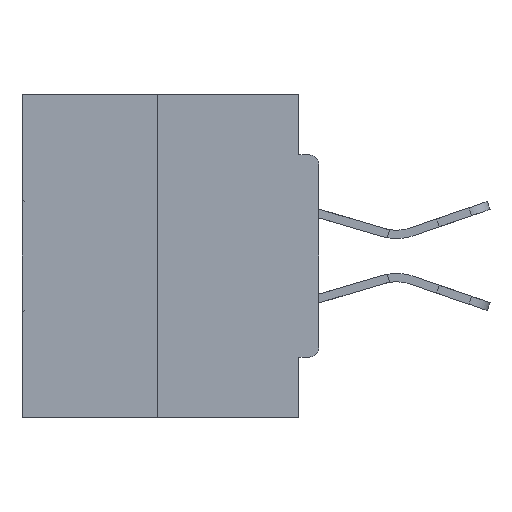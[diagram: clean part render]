
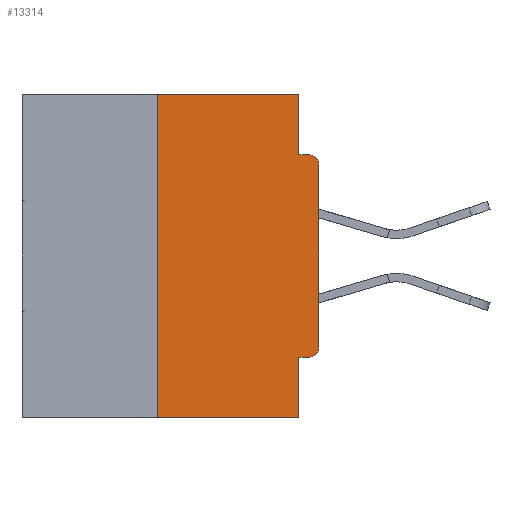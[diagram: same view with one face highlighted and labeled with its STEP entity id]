
A CAD part, left-side view. The second image highlights one B-rep face of the part: STEP entity #13314.
In plain terms, the highlighted planar face has unit normal (-1, 0, 0).
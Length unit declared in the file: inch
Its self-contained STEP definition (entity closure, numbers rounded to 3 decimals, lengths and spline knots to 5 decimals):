
#20 = PLANE ( 'NONE',  #43346 ) ;
#307 = CARTESIAN_POINT ( 'NONE',  ( 0., 0., -0.1085 ) ) ;
#514 = CARTESIAN_POINT ( 'NONE',  ( 0., 0.031, -0.4065 ) ) ;
#758 = ORIENTED_EDGE ( 'NONE', *, *, #14378, .F. ) ;
#1119 = VERTEX_POINT ( 'NONE', #307 ) ;
#1191 = EDGE_CURVE ( 'NONE', #15538, #8642, #17899, .T. ) ;
#1351 = LINE ( 'NONE', #39865, #3982 ) ;
#1389 = CARTESIAN_POINT ( 'NONE',  ( 0., 0.031, 0. ) ) ;
#2072 = LINE ( 'NONE', #3896, #15142 ) ;
#3095 = VECTOR ( 'NONE', #6852, 39.37008 ) ;
#3896 = CARTESIAN_POINT ( 'NONE',  ( 0., 0., -0.4065 ) ) ;
#3982 = VECTOR ( 'NONE', #26684, 39.37008 ) ;
#5141 = FACE_OUTER_BOUND ( 'NONE', #34798, .T. ) ;
#5734 = ORIENTED_EDGE ( 'NONE', *, *, #24932, .T. ) ;
#5832 = LINE ( 'NONE', #37845, #40338 ) ;
#6600 = CARTESIAN_POINT ( 'NONE',  ( 0., 0.031, -0.0935 ) ) ;
#6852 = DIRECTION ( 'NONE',  ( 0., 0., 1. ) ) ;
#8642 = VERTEX_POINT ( 'NONE', #16960 ) ;
#9210 = ORIENTED_EDGE ( 'NONE', *, *, #31386, .F. ) ;
#9304 = CARTESIAN_POINT ( 'NONE',  ( 0., 0., -0.0935 ) ) ;
#11231 = DIRECTION ( 'NONE',  ( 0., 0., -1. ) ) ;
#12776 = EDGE_CURVE ( 'NONE', #22746, #1119, #30275, .T. ) ;
#13314 = ADVANCED_FACE ( 'NONE', ( #5141 ), #20, .F. ) ;
#13691 = LINE ( 'NONE', #14069, #20993 ) ;
#14069 = CARTESIAN_POINT ( 'NONE',  ( 0., 0.25, 0. ) ) ;
#14216 = CARTESIAN_POINT ( 'NONE',  ( 0., 0.015, -0.4065 ) ) ;
#14378 = EDGE_CURVE ( 'NONE', #21782, #18243, #1351, .T. ) ;
#15142 = VECTOR ( 'NONE', #37388, 39.37008 ) ;
#15211 = CARTESIAN_POINT ( 'NONE',  ( 0., 0.25, -0.5 ) ) ;
#15538 = VERTEX_POINT ( 'NONE', #15211 ) ;
#15846 = ORIENTED_EDGE ( 'NONE', *, *, #1191, .T. ) ;
#15968 = CARTESIAN_POINT ( 'NONE',  ( 0., 0.015, -0.3915 ) ) ;
#16436 = CARTESIAN_POINT ( 'NONE',  ( 0., 0.015, -0.1085 ) ) ;
#16960 = CARTESIAN_POINT ( 'NONE',  ( 0., 0.031, -0.5 ) ) ;
#17398 = DIRECTION ( 'NONE',  ( 0., 0., 1. ) ) ;
#17876 = ORIENTED_EDGE ( 'NONE', *, *, #18327, .F. ) ;
#17899 = LINE ( 'NONE', #40274, #33579 ) ;
#18243 = VERTEX_POINT ( 'NONE', #41948 ) ;
#18327 = EDGE_CURVE ( 'NONE', #23149, #32677, #31568, .T. ) ;
#19325 = DIRECTION ( 'NONE',  ( -1., 0., 0. ) ) ;
#19808 = DIRECTION ( 'NONE',  ( 0., 0., -1. ) ) ;
#20993 = VECTOR ( 'NONE', #17398, 39.37008 ) ;
#21192 = CARTESIAN_POINT ( 'NONE',  ( 0., 0.25, 0. ) ) ;
#21782 = VERTEX_POINT ( 'NONE', #21192 ) ;
#22010 = AXIS2_PLACEMENT_3D ( 'NONE', #16436, #35870, #36016 ) ;
#22607 = CARTESIAN_POINT ( 'NONE',  ( 0., 0., 0. ) ) ;
#22614 = VECTOR ( 'NONE', #32389, 39.37008 ) ;
#22663 = DIRECTION ( 'NONE',  ( 0., 0., -1. ) ) ;
#22746 = VERTEX_POINT ( 'NONE', #40849 ) ;
#23149 = VERTEX_POINT ( 'NONE', #6600 ) ;
#24032 = ORIENTED_EDGE ( 'NONE', *, *, #43118, .F. ) ;
#24269 = ORIENTED_EDGE ( 'NONE', *, *, #26075, .F. ) ;
#24932 = EDGE_CURVE ( 'NONE', #30819, #22746, #27378, .T. ) ;
#26075 = EDGE_CURVE ( 'NONE', #15538, #21782, #13691, .T. ) ;
#26552 = AXIS2_PLACEMENT_3D ( 'NONE', #15968, #19325, #22663 ) ;
#26684 = DIRECTION ( 'NONE',  ( 0., -1., 0. ) ) ;
#26820 = DIRECTION ( 'NONE',  ( 1., 0., 0. ) ) ;
#26928 = ORIENTED_EDGE ( 'NONE', *, *, #43078, .T. ) ;
#27101 = ORIENTED_EDGE ( 'NONE', *, *, #38240, .F. ) ;
#27378 = CIRCLE ( 'NONE', #26552, 0.015 ) ;
#29883 = CARTESIAN_POINT ( 'NONE',  ( 0., 0.46, 0. ) ) ;
#30123 = VECTOR ( 'NONE', #11231, 39.37008 ) ;
#30275 = LINE ( 'NONE', #22607, #3095 ) ;
#30819 = VERTEX_POINT ( 'NONE', #14216 ) ;
#31386 = EDGE_CURVE ( 'NONE', #18243, #23149, #32759, .T. ) ;
#31568 = LINE ( 'NONE', #9304, #22614 ) ;
#32389 = DIRECTION ( 'NONE',  ( 0., -1., 0. ) ) ;
#32677 = VERTEX_POINT ( 'NONE', #40382 ) ;
#32759 = LINE ( 'NONE', #1389, #30123 ) ;
#32955 = VERTEX_POINT ( 'NONE', #514 ) ;
#33196 = DIRECTION ( 'NONE',  ( 0., 0., -1. ) ) ;
#33579 = VECTOR ( 'NONE', #37329, 39.37008 ) ;
#33884 = ORIENTED_EDGE ( 'NONE', *, *, #12776, .T. ) ;
#34798 = EDGE_LOOP ( 'NONE', ( #758, #24269, #15846, #24032, #27101, #5734, #33884, #26928, #17876, #9210 ) ) ;
#35870 = DIRECTION ( 'NONE',  ( -1., 0., 0. ) ) ;
#36016 = DIRECTION ( 'NONE',  ( 0., 0., -1. ) ) ;
#36131 = CIRCLE ( 'NONE', #22010, 0.015 ) ;
#37329 = DIRECTION ( 'NONE',  ( 0., -1., 0. ) ) ;
#37388 = DIRECTION ( 'NONE',  ( 0., 1., 0. ) ) ;
#37845 = CARTESIAN_POINT ( 'NONE',  ( 0., 0.031, -0.5 ) ) ;
#38240 = EDGE_CURVE ( 'NONE', #30819, #32955, #2072, .T. ) ;
#39865 = CARTESIAN_POINT ( 'NONE',  ( 0., 0.46, 0. ) ) ;
#40274 = CARTESIAN_POINT ( 'NONE',  ( 0., 0.46, -0.5 ) ) ;
#40338 = VECTOR ( 'NONE', #33196, 39.37008 ) ;
#40382 = CARTESIAN_POINT ( 'NONE',  ( 0., 0.015, -0.0935 ) ) ;
#40849 = CARTESIAN_POINT ( 'NONE',  ( 0., 0., -0.3915 ) ) ;
#41948 = CARTESIAN_POINT ( 'NONE',  ( 0., 0.031, 0. ) ) ;
#43078 = EDGE_CURVE ( 'NONE', #1119, #32677, #36131, .T. ) ;
#43118 = EDGE_CURVE ( 'NONE', #32955, #8642, #5832, .T. ) ;
#43346 = AXIS2_PLACEMENT_3D ( 'NONE', #29883, #26820, #19808 ) ;
